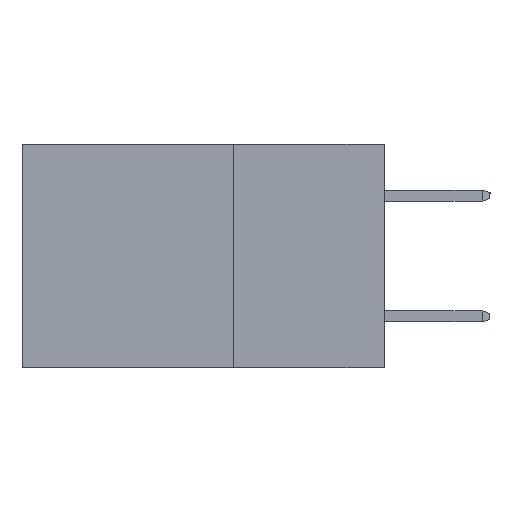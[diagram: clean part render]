
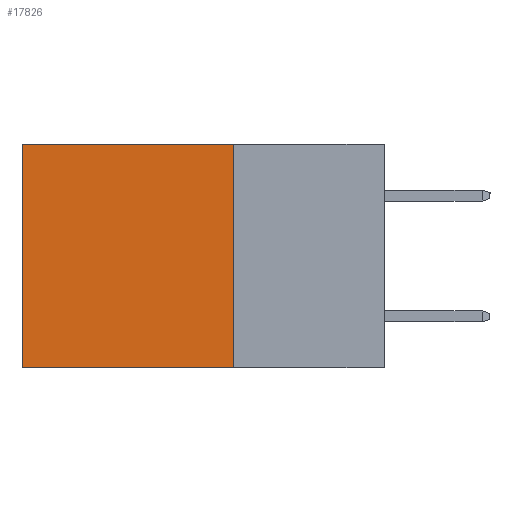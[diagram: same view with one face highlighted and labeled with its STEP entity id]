
A CAD part, left-side view. The second image highlights one B-rep face of the part: STEP entity #17826.
In plain terms, the highlighted planar face has unit normal (-1, 0, 0).
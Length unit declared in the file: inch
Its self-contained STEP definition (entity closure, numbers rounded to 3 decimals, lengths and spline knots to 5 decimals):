
#224 = CARTESIAN_POINT ( 'NONE',  ( 0.2615, 0.6, -0.37 ) ) ;
#322 = EDGE_CURVE ( 'NONE', #13172, #16335, #18969, .T. ) ;
#3976 = LINE ( 'NONE', #12415, #20311 ) ;
#4646 = CARTESIAN_POINT ( 'NONE',  ( 0.2615, 0.6, -0.37 ) ) ;
#5508 = CARTESIAN_POINT ( 'NONE',  ( 0.2615, 0.25, -0.37 ) ) ;
#5980 = DIRECTION ( 'NONE',  ( 0., 0., -1. ) ) ;
#6021 = EDGE_CURVE ( 'NONE', #21115, #6272, #21883, .T. ) ;
#6272 = VERTEX_POINT ( 'NONE', #11069 ) ;
#7189 = ORIENTED_EDGE ( 'NONE', *, *, #6021, .T. ) ;
#7871 = DIRECTION ( 'NONE',  ( 1., 0., 0. ) ) ;
#8040 = VECTOR ( 'NONE', #12286, 39.37008 ) ;
#8928 = VECTOR ( 'NONE', #9775, 39.37008 ) ;
#9658 = LINE ( 'NONE', #4646, #8928 ) ;
#9775 = DIRECTION ( 'NONE',  ( 0., 0., -1. ) ) ;
#11069 = CARTESIAN_POINT ( 'NONE',  ( 0.2615, 0.6, 0. ) ) ;
#12116 = AXIS2_PLACEMENT_3D ( 'NONE', #19454, #7871, #5980 ) ;
#12286 = DIRECTION ( 'NONE',  ( 0., 1., 0. ) ) ;
#12415 = CARTESIAN_POINT ( 'NONE',  ( 0.2615, 0.25, -0.37 ) ) ;
#13075 = EDGE_LOOP ( 'NONE', ( #14510, #15419, #17897, #7189 ) ) ;
#13172 = VERTEX_POINT ( 'NONE', #20488 ) ;
#14510 = ORIENTED_EDGE ( 'NONE', *, *, #17866, .T. ) ;
#15390 = VECTOR ( 'NONE', #18529, 39.37008 ) ;
#15419 = ORIENTED_EDGE ( 'NONE', *, *, #322, .F. ) ;
#15526 = DIRECTION ( 'NONE',  ( 0., 0., -1. ) ) ;
#16326 = PLANE ( 'NONE',  #12116 ) ;
#16335 = VERTEX_POINT ( 'NONE', #224 ) ;
#17826 = ADVANCED_FACE ( 'NONE', ( #21339 ), #16326, .F. ) ;
#17866 = EDGE_CURVE ( 'NONE', #6272, #16335, #9658, .T. ) ;
#17897 = ORIENTED_EDGE ( 'NONE', *, *, #18535, .F. ) ;
#18529 = DIRECTION ( 'NONE',  ( 0., 1., 0. ) ) ;
#18535 = EDGE_CURVE ( 'NONE', #21115, #13172, #3976, .T. ) ;
#18969 = LINE ( 'NONE', #5508, #8040 ) ;
#19454 = CARTESIAN_POINT ( 'NONE',  ( 0.2615, 0.25, -0.37 ) ) ;
#20296 = CARTESIAN_POINT ( 'NONE',  ( 0.2615, 0.25, 0. ) ) ;
#20311 = VECTOR ( 'NONE', #15526, 39.37008 ) ;
#20488 = CARTESIAN_POINT ( 'NONE',  ( 0.2615, 0.25, -0.37 ) ) ;
#21115 = VERTEX_POINT ( 'NONE', #20296 ) ;
#21339 = FACE_OUTER_BOUND ( 'NONE', #13075, .T. ) ;
#21768 = CARTESIAN_POINT ( 'NONE',  ( 0.2615, 0.25, 0. ) ) ;
#21883 = LINE ( 'NONE', #21768, #15390 ) ;
